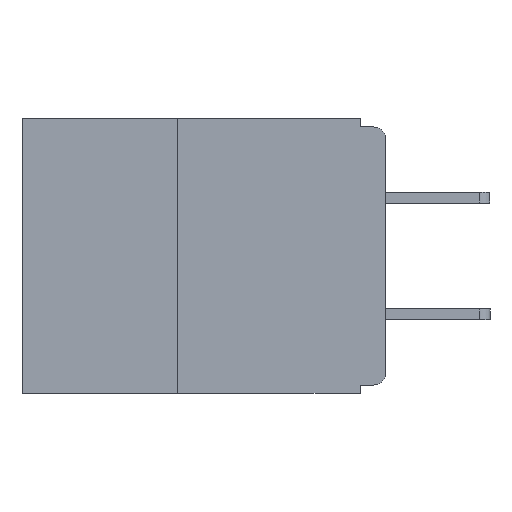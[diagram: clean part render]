
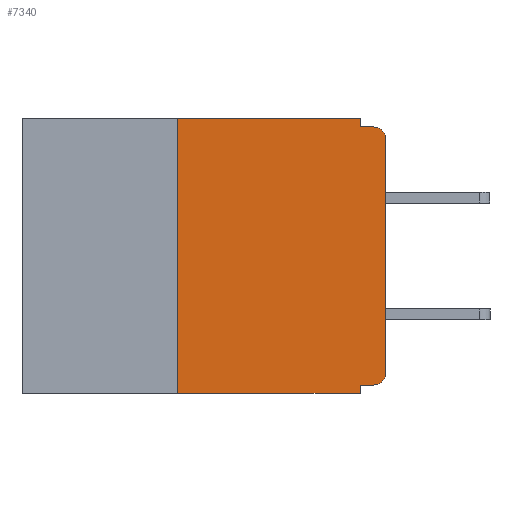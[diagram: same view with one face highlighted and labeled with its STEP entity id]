
A CAD part, left-side view. The second image highlights one B-rep face of the part: STEP entity #7340.
In plain terms, the highlighted planar face has unit normal (-1, 0, 0).
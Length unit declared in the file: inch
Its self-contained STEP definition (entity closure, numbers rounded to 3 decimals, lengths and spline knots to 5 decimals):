
#24 = CIRCLE ( 'NONE', #9585, 0.015 ) ;
#452 = CARTESIAN_POINT ( 'NONE',  ( 0., 0.015, -0.32 ) ) ;
#860 = CIRCLE ( 'NONE', #18517, 0.015 ) ;
#925 = ORIENTED_EDGE ( 'NONE', *, *, #12067, .F. ) ;
#1037 = CARTESIAN_POINT ( 'NONE',  ( 0., 0.031, 0. ) ) ;
#2190 = CARTESIAN_POINT ( 'NONE',  ( 0., 0., -0.32 ) ) ;
#2791 = ORIENTED_EDGE ( 'NONE', *, *, #11241, .T. ) ;
#3314 = LINE ( 'NONE', #11426, #11100 ) ;
#3705 = DIRECTION ( 'NONE',  ( 0., 1., 0. ) ) ;
#4188 = ORIENTED_EDGE ( 'NONE', *, *, #5672, .F. ) ;
#4210 = ORIENTED_EDGE ( 'NONE', *, *, #17030, .T. ) ;
#4324 = VERTEX_POINT ( 'NONE', #18293 ) ;
#4471 = CARTESIAN_POINT ( 'NONE',  ( 0., 0.25, -0.33 ) ) ;
#4694 = DIRECTION ( 'NONE',  ( 0., -1., 0. ) ) ;
#4755 = VERTEX_POINT ( 'NONE', #10511 ) ;
#4820 = DIRECTION ( 'NONE',  ( -1., 0., 0. ) ) ;
#4997 = VECTOR ( 'NONE', #12529, 39.37008 ) ;
#5084 = DIRECTION ( 'NONE',  ( 0., -1., 0. ) ) ;
#5146 = VERTEX_POINT ( 'NONE', #17528 ) ;
#5245 = CARTESIAN_POINT ( 'NONE',  ( 0., 0.437, 0. ) ) ;
#5364 = DIRECTION ( 'NONE',  ( 0., 0., -1. ) ) ;
#5368 = DIRECTION ( 'NONE',  ( 1., 0., 0. ) ) ;
#5427 = PLANE ( 'NONE',  #18100 ) ;
#5465 = LINE ( 'NONE', #13951, #4997 ) ;
#5614 = CARTESIAN_POINT ( 'NONE',  ( 0., 0.437, 0. ) ) ;
#5672 = EDGE_CURVE ( 'NONE', #5146, #6439, #9075, .T. ) ;
#5964 = VECTOR ( 'NONE', #6941, 39.37008 ) ;
#6023 = ORIENTED_EDGE ( 'NONE', *, *, #17256, .F. ) ;
#6439 = VERTEX_POINT ( 'NONE', #13567 ) ;
#6680 = EDGE_CURVE ( 'NONE', #7137, #15076, #3314, .T. ) ;
#6793 = VERTEX_POINT ( 'NONE', #10436 ) ;
#6941 = DIRECTION ( 'NONE',  ( 0., 0., -1. ) ) ;
#7137 = VERTEX_POINT ( 'NONE', #7557 ) ;
#7340 = ADVANCED_FACE ( 'NONE', ( #7859 ), #5427, .F. ) ;
#7387 = VECTOR ( 'NONE', #3705, 39.37008 ) ;
#7557 = CARTESIAN_POINT ( 'NONE',  ( 0., 0., -0.305 ) ) ;
#7572 = LINE ( 'NONE', #4471, #18372 ) ;
#7859 = FACE_OUTER_BOUND ( 'NONE', #9684, .T. ) ;
#7884 = VERTEX_POINT ( 'NONE', #452 ) ;
#8405 = EDGE_CURVE ( 'NONE', #6439, #4324, #13247, .T. ) ;
#8421 = DIRECTION ( 'NONE',  ( -1., 0., 0. ) ) ;
#8611 = VECTOR ( 'NONE', #5084, 39.37008 ) ;
#8731 = DIRECTION ( 'NONE',  ( 0., -1., 0. ) ) ;
#9075 = LINE ( 'NONE', #5245, #8611 ) ;
#9223 = CARTESIAN_POINT ( 'NONE',  ( 0., 0., -0.025 ) ) ;
#9585 = AXIS2_PLACEMENT_3D ( 'NONE', #13537, #4820, #14951 ) ;
#9684 = EDGE_LOOP ( 'NONE', ( #17798, #2791, #18413, #14831, #4188, #6023, #10393, #925, #13989, #4210 ) ) ;
#10353 = EDGE_CURVE ( 'NONE', #6793, #13615, #10957, .T. ) ;
#10393 = ORIENTED_EDGE ( 'NONE', *, *, #10353, .T. ) ;
#10436 = CARTESIAN_POINT ( 'NONE',  ( 0., 0.25, -0.33 ) ) ;
#10511 = CARTESIAN_POINT ( 'NONE',  ( 0., 0.015, -0.01 ) ) ;
#10589 = CARTESIAN_POINT ( 'NONE',  ( 0., 0.031, -0.33 ) ) ;
#10957 = LINE ( 'NONE', #17190, #18320 ) ;
#11100 = VECTOR ( 'NONE', #11312, 39.37008 ) ;
#11241 = EDGE_CURVE ( 'NONE', #15076, #4755, #24, .T. ) ;
#11312 = DIRECTION ( 'NONE',  ( 0., 0., 1. ) ) ;
#11426 = CARTESIAN_POINT ( 'NONE',  ( 0., 0., 0. ) ) ;
#12067 = EDGE_CURVE ( 'NONE', #12972, #13615, #5465, .T. ) ;
#12286 = LINE ( 'NONE', #14821, #16010 ) ;
#12529 = DIRECTION ( 'NONE',  ( 0., 0., -1. ) ) ;
#12972 = VERTEX_POINT ( 'NONE', #14752 ) ;
#12990 = EDGE_CURVE ( 'NONE', #4324, #4755, #12286, .T. ) ;
#13199 = DIRECTION ( 'NONE',  ( 0., 0., 1. ) ) ;
#13247 = LINE ( 'NONE', #1037, #5964 ) ;
#13537 = CARTESIAN_POINT ( 'NONE',  ( 0., 0.015, -0.025 ) ) ;
#13567 = CARTESIAN_POINT ( 'NONE',  ( 0., 0.031, 0. ) ) ;
#13615 = VERTEX_POINT ( 'NONE', #10589 ) ;
#13951 = CARTESIAN_POINT ( 'NONE',  ( 0., 0.031, -0.33 ) ) ;
#13989 = ORIENTED_EDGE ( 'NONE', *, *, #15211, .F. ) ;
#14752 = CARTESIAN_POINT ( 'NONE',  ( 0., 0.031, -0.32 ) ) ;
#14821 = CARTESIAN_POINT ( 'NONE',  ( 0., 0., -0.01 ) ) ;
#14831 = ORIENTED_EDGE ( 'NONE', *, *, #8405, .F. ) ;
#14951 = DIRECTION ( 'NONE',  ( 0., 0., -1. ) ) ;
#15058 = LINE ( 'NONE', #2190, #7387 ) ;
#15076 = VERTEX_POINT ( 'NONE', #9223 ) ;
#15211 = EDGE_CURVE ( 'NONE', #7884, #12972, #15058, .T. ) ;
#16010 = VECTOR ( 'NONE', #4694, 39.37008 ) ;
#16905 = CARTESIAN_POINT ( 'NONE',  ( 0., 0.015, -0.305 ) ) ;
#17030 = EDGE_CURVE ( 'NONE', #7884, #7137, #860, .T. ) ;
#17190 = CARTESIAN_POINT ( 'NONE',  ( 0., 0.437, -0.33 ) ) ;
#17256 = EDGE_CURVE ( 'NONE', #6793, #5146, #7572, .T. ) ;
#17528 = CARTESIAN_POINT ( 'NONE',  ( 0., 0.25, 0. ) ) ;
#17798 = ORIENTED_EDGE ( 'NONE', *, *, #6680, .T. ) ;
#18100 = AXIS2_PLACEMENT_3D ( 'NONE', #5614, #5368, #5364 ) ;
#18252 = DIRECTION ( 'NONE',  ( 0., 0., -1. ) ) ;
#18293 = CARTESIAN_POINT ( 'NONE',  ( 0., 0.031, -0.01 ) ) ;
#18320 = VECTOR ( 'NONE', #8731, 39.37008 ) ;
#18372 = VECTOR ( 'NONE', #13199, 39.37008 ) ;
#18413 = ORIENTED_EDGE ( 'NONE', *, *, #12990, .F. ) ;
#18517 = AXIS2_PLACEMENT_3D ( 'NONE', #16905, #8421, #18252 ) ;
